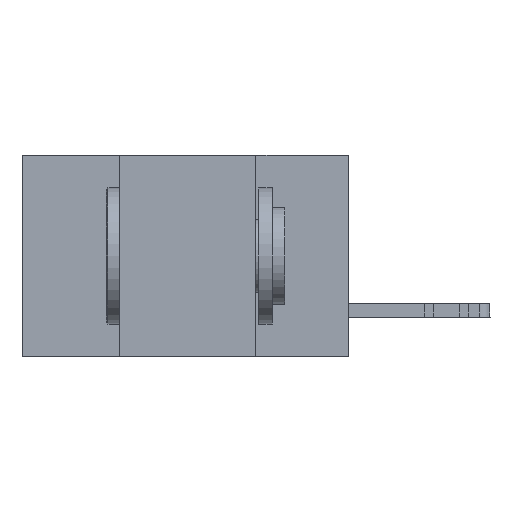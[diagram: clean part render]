
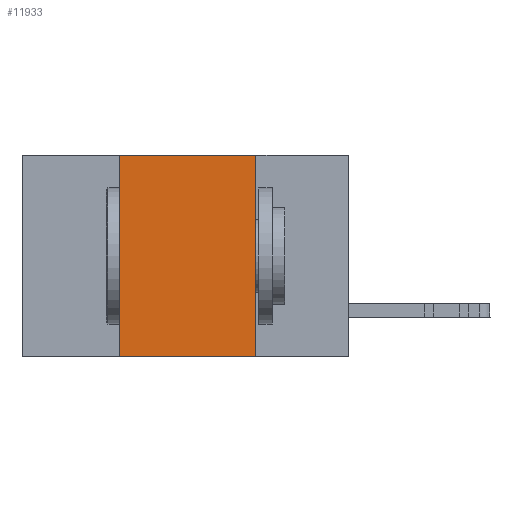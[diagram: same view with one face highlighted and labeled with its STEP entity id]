
A CAD part, left-side view. The second image highlights one B-rep face of the part: STEP entity #11933.
In plain terms, the highlighted planar face has unit normal (-1, 0, 0).
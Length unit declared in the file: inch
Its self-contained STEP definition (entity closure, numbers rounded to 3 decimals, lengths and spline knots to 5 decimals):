
#439 = LINE ( 'NONE', #24922, #24842 ) ;
#2085 = DIRECTION ( 'NONE',  ( 0., -1., 0. ) ) ;
#3349 = AXIS2_PLACEMENT_3D ( 'NONE', #28248, #26151, #26292 ) ;
#3371 = ORIENTED_EDGE ( 'NONE', *, *, #18115, .T. ) ;
#5717 = PLANE ( 'NONE',  #3349 ) ;
#6315 = VECTOR ( 'NONE', #26002, 39.37008 ) ;
#6432 = LINE ( 'NONE', #8366, #15003 ) ;
#7534 = LINE ( 'NONE', #19007, #6315 ) ;
#8366 = CARTESIAN_POINT ( 'NONE',  ( 0., 0.6, -0.37 ) ) ;
#8973 = CARTESIAN_POINT ( 'NONE',  ( 0., 0.42, -0.37 ) ) ;
#9285 = CARTESIAN_POINT ( 'NONE',  ( 0., 0.42, 0. ) ) ;
#11509 = LINE ( 'NONE', #9285, #27947 ) ;
#11933 = ADVANCED_FACE ( 'NONE', ( #12730 ), #5717, .F. ) ;
#12623 = EDGE_CURVE ( 'NONE', #19100, #23956, #439, .T. ) ;
#12730 = FACE_OUTER_BOUND ( 'NONE', #20498, .T. ) ;
#13952 = VERTEX_POINT ( 'NONE', #8973 ) ;
#14918 = ORIENTED_EDGE ( 'NONE', *, *, #26696, .F. ) ;
#15003 = VECTOR ( 'NONE', #2085, 39.37008 ) ;
#15152 = CARTESIAN_POINT ( 'NONE',  ( 0., 0.42, 0. ) ) ;
#15459 = ORIENTED_EDGE ( 'NONE', *, *, #19358, .F. ) ;
#15678 = DIRECTION ( 'NONE',  ( 0., -1., 0. ) ) ;
#16860 = CARTESIAN_POINT ( 'NONE',  ( 0., 0.17, 0. ) ) ;
#18087 = DIRECTION ( 'NONE',  ( 0., 0., 1. ) ) ;
#18115 = EDGE_CURVE ( 'NONE', #13952, #18909, #6432, .T. ) ;
#18909 = VERTEX_POINT ( 'NONE', #21119 ) ;
#19007 = CARTESIAN_POINT ( 'NONE',  ( 0., 0.17, 0. ) ) ;
#19100 = VERTEX_POINT ( 'NONE', #15152 ) ;
#19358 = EDGE_CURVE ( 'NONE', #23956, #18909, #7534, .T. ) ;
#20498 = EDGE_LOOP ( 'NONE', ( #15459, #25245, #14918, #3371 ) ) ;
#21119 = CARTESIAN_POINT ( 'NONE',  ( 0., 0.17, -0.37 ) ) ;
#23956 = VERTEX_POINT ( 'NONE', #16860 ) ;
#24842 = VECTOR ( 'NONE', #15678, 39.37008 ) ;
#24922 = CARTESIAN_POINT ( 'NONE',  ( 0., 0.6, 0. ) ) ;
#25245 = ORIENTED_EDGE ( 'NONE', *, *, #12623, .F. ) ;
#26002 = DIRECTION ( 'NONE',  ( 0., 0., -1. ) ) ;
#26151 = DIRECTION ( 'NONE',  ( 1., 0., 0. ) ) ;
#26292 = DIRECTION ( 'NONE',  ( 0., 0., -1. ) ) ;
#26696 = EDGE_CURVE ( 'NONE', #13952, #19100, #11509, .T. ) ;
#27947 = VECTOR ( 'NONE', #18087, 39.37008 ) ;
#28248 = CARTESIAN_POINT ( 'NONE',  ( 0., 0.6, 0. ) ) ;
